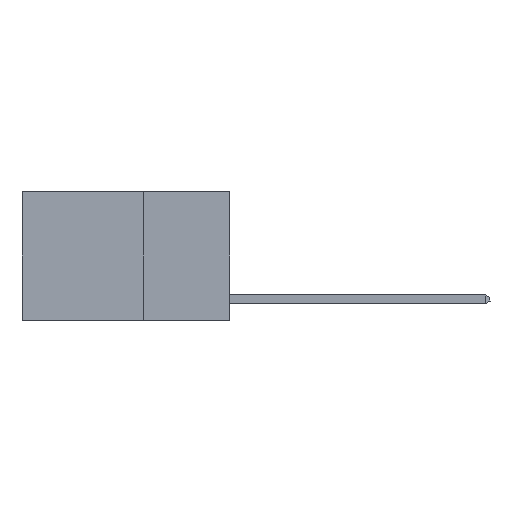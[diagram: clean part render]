
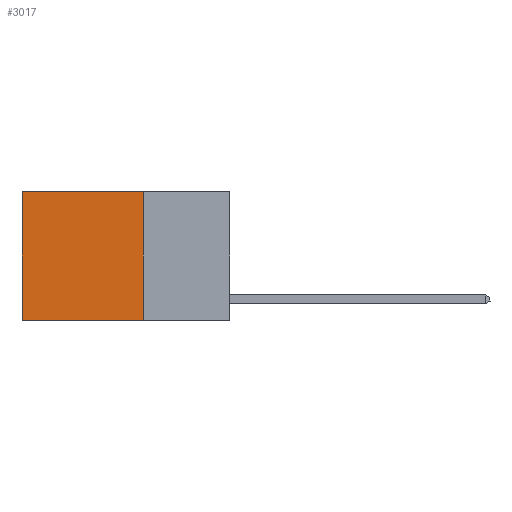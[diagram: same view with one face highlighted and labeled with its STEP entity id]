
A CAD part, left-side view. The second image highlights one B-rep face of the part: STEP entity #3017.
In plain terms, the highlighted planar face has unit normal (-1, 0, 0).
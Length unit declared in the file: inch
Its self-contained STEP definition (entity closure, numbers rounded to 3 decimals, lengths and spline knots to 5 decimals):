
#81 = DIRECTION ( 'NONE',  ( 0., 0., -1. ) ) ;
#1102 = PLANE ( 'NONE',  #6041 ) ;
#1148 = CARTESIAN_POINT ( 'NONE',  ( 0.2625, 0.6, 0. ) ) ;
#1201 = EDGE_CURVE ( 'NONE', #7896, #11067, #9888, .T. ) ;
#1535 = CARTESIAN_POINT ( 'NONE',  ( 0.2625, 0.25, 0. ) ) ;
#1887 = CARTESIAN_POINT ( 'NONE',  ( 0.2625, 0.6, 0. ) ) ;
#1907 = VECTOR ( 'NONE', #13337, 39.37008 ) ;
#2350 = ORIENTED_EDGE ( 'NONE', *, *, #1201, .F. ) ;
#2640 = CARTESIAN_POINT ( 'NONE',  ( 0.2625, 0.25, 0. ) ) ;
#2832 = ORIENTED_EDGE ( 'NONE', *, *, #6450, .T. ) ;
#3017 = ADVANCED_FACE ( 'NONE', ( #12143 ), #1102, .F. ) ;
#3271 = DIRECTION ( 'NONE',  ( 1., 0., 0. ) ) ;
#4024 = VECTOR ( 'NONE', #7921, 39.37008 ) ;
#4268 = CARTESIAN_POINT ( 'NONE',  ( 0.2625, 0.25, 0. ) ) ;
#4489 = DIRECTION ( 'NONE',  ( 0., 0., -1. ) ) ;
#4845 = VECTOR ( 'NONE', #81, 39.37008 ) ;
#5503 = ORIENTED_EDGE ( 'NONE', *, *, #11031, .F. ) ;
#5693 = LINE ( 'NONE', #2640, #4024 ) ;
#5860 = EDGE_LOOP ( 'NONE', ( #6478, #2350, #5503, #2832 ) ) ;
#6041 = AXIS2_PLACEMENT_3D ( 'NONE', #4268, #3271, #4489 ) ;
#6450 = EDGE_CURVE ( 'NONE', #9558, #11206, #9111, .T. ) ;
#6478 = ORIENTED_EDGE ( 'NONE', *, *, #8691, .T. ) ;
#6583 = DIRECTION ( 'NONE',  ( 0., 1., 0. ) ) ;
#6603 = LINE ( 'NONE', #1148, #4845 ) ;
#7279 = VECTOR ( 'NONE', #6583, 39.37008 ) ;
#7896 = VERTEX_POINT ( 'NONE', #9062 ) ;
#7921 = DIRECTION ( 'NONE',  ( 0., 0., -1. ) ) ;
#8691 = EDGE_CURVE ( 'NONE', #11206, #11067, #6603, .T. ) ;
#9062 = CARTESIAN_POINT ( 'NONE',  ( 0.2625, 0.25, -0.37 ) ) ;
#9111 = LINE ( 'NONE', #1535, #7279 ) ;
#9558 = VERTEX_POINT ( 'NONE', #9992 ) ;
#9888 = LINE ( 'NONE', #13058, #1907 ) ;
#9992 = CARTESIAN_POINT ( 'NONE',  ( 0.2625, 0.25, 0. ) ) ;
#11031 = EDGE_CURVE ( 'NONE', #9558, #7896, #5693, .T. ) ;
#11067 = VERTEX_POINT ( 'NONE', #11279 ) ;
#11206 = VERTEX_POINT ( 'NONE', #1887 ) ;
#11279 = CARTESIAN_POINT ( 'NONE',  ( 0.2625, 0.6, -0.37 ) ) ;
#12143 = FACE_OUTER_BOUND ( 'NONE', #5860, .T. ) ;
#13058 = CARTESIAN_POINT ( 'NONE',  ( 0.2625, 0.25, -0.37 ) ) ;
#13337 = DIRECTION ( 'NONE',  ( 0., 1., 0. ) ) ;
